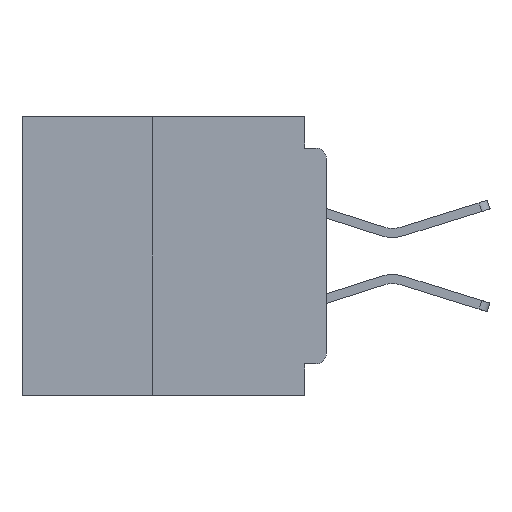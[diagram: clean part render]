
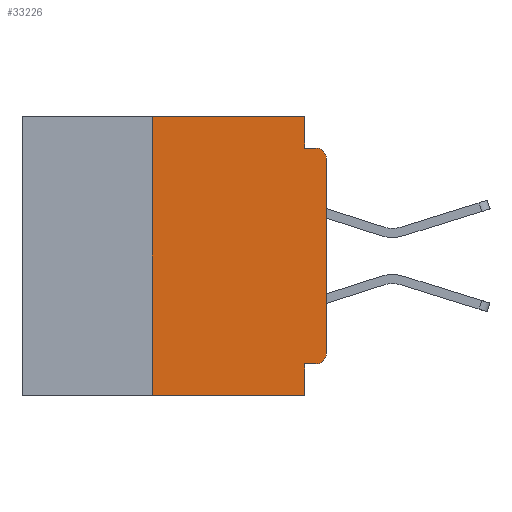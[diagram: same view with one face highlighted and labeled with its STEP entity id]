
A CAD part, left-side view. The second image highlights one B-rep face of the part: STEP entity #33226.
In plain terms, the highlighted planar face has unit normal (-1, 0, 0).
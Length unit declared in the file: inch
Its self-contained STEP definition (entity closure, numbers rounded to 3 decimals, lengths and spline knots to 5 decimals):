
#401 = DIRECTION ( 'NONE',  ( 0., -1., 0. ) ) ;
#425 = CARTESIAN_POINT ( 'NONE',  ( 0., 0., -0.06 ) ) ;
#578 = ORIENTED_EDGE ( 'NONE', *, *, #38165, .F. ) ;
#789 = VECTOR ( 'NONE', #48759, 39.37008 ) ;
#852 = VECTOR ( 'NONE', #14999, 39.37008 ) ;
#1643 = CARTESIAN_POINT ( 'NONE',  ( 0., 0.437, 0. ) ) ;
#2049 = CARTESIAN_POINT ( 'NONE',  ( 0., 0.031, -0.4 ) ) ;
#2297 = VECTOR ( 'NONE', #5242, 39.37008 ) ;
#2617 = CIRCLE ( 'NONE', #19181, 0.015 ) ;
#2740 = ORIENTED_EDGE ( 'NONE', *, *, #18805, .F. ) ;
#3304 = VECTOR ( 'NONE', #26643, 39.37008 ) ;
#3781 = LINE ( 'NONE', #22472, #22875 ) ;
#4065 = EDGE_CURVE ( 'NONE', #16272, #38870, #24792, .T. ) ;
#5242 = DIRECTION ( 'NONE',  ( 0., 0., 1. ) ) ;
#5841 = ORIENTED_EDGE ( 'NONE', *, *, #9505, .T. ) ;
#8282 = EDGE_CURVE ( 'NONE', #13142, #38329, #22589, .T. ) ;
#8519 = VERTEX_POINT ( 'NONE', #48036 ) ;
#9505 = EDGE_CURVE ( 'NONE', #8519, #13142, #39668, .T. ) ;
#10257 = VERTEX_POINT ( 'NONE', #2049 ) ;
#11177 = VECTOR ( 'NONE', #35939, 39.37008 ) ;
#11187 = ORIENTED_EDGE ( 'NONE', *, *, #14609, .T. ) ;
#11631 = VERTEX_POINT ( 'NONE', #39704 ) ;
#12135 = VERTEX_POINT ( 'NONE', #31903 ) ;
#12309 = VERTEX_POINT ( 'NONE', #13692 ) ;
#13142 = VERTEX_POINT ( 'NONE', #18499 ) ;
#13692 = CARTESIAN_POINT ( 'NONE',  ( 0., 0.25, -0.4 ) ) ;
#13794 = CARTESIAN_POINT ( 'NONE',  ( 0., 0.015, -0.06 ) ) ;
#14436 = ORIENTED_EDGE ( 'NONE', *, *, #41662, .F. ) ;
#14609 = EDGE_CURVE ( 'NONE', #38329, #15548, #2617, .T. ) ;
#14853 = CARTESIAN_POINT ( 'NONE',  ( 0., 0.031, -0.045 ) ) ;
#14999 = DIRECTION ( 'NONE',  ( 0., 1., 0. ) ) ;
#15255 = ORIENTED_EDGE ( 'NONE', *, *, #32517, .F. ) ;
#15407 = CARTESIAN_POINT ( 'NONE',  ( 0., 0.015, -0.045 ) ) ;
#15548 = VERTEX_POINT ( 'NONE', #15407 ) ;
#15717 = CARTESIAN_POINT ( 'NONE',  ( 0., 0., -0.045 ) ) ;
#16272 = VERTEX_POINT ( 'NONE', #19513 ) ;
#17672 = DIRECTION ( 'NONE',  ( 0., 0., -1. ) ) ;
#18499 = CARTESIAN_POINT ( 'NONE',  ( 0., 0., -0.34 ) ) ;
#18805 = EDGE_CURVE ( 'NONE', #38870, #15548, #45059, .T. ) ;
#19181 = AXIS2_PLACEMENT_3D ( 'NONE', #13794, #40403, #17672 ) ;
#19513 = CARTESIAN_POINT ( 'NONE',  ( 0., 0.031, 0. ) ) ;
#19875 = LINE ( 'NONE', #44783, #789 ) ;
#20286 = DIRECTION ( 'NONE',  ( -1., 0., 0. ) ) ;
#20935 = EDGE_LOOP ( 'NONE', ( #47976, #11187, #2740, #35956, #14436, #578, #30535, #21364, #15255, #5841 ) ) ;
#21364 = ORIENTED_EDGE ( 'NONE', *, *, #33105, .F. ) ;
#21373 = LINE ( 'NONE', #1643, #11177 ) ;
#22472 = CARTESIAN_POINT ( 'NONE',  ( 0., 0.031, -0.4 ) ) ;
#22529 = CARTESIAN_POINT ( 'NONE',  ( 0., 0., -0.355 ) ) ;
#22589 = LINE ( 'NONE', #35703, #2297 ) ;
#22875 = VECTOR ( 'NONE', #41374, 39.37008 ) ;
#23727 = CARTESIAN_POINT ( 'NONE',  ( 0., 0.437, -0.4 ) ) ;
#24792 = LINE ( 'NONE', #26522, #3304 ) ;
#26522 = CARTESIAN_POINT ( 'NONE',  ( 0., 0.031, 0. ) ) ;
#26643 = DIRECTION ( 'NONE',  ( 0., 0., -1. ) ) ;
#27132 = CARTESIAN_POINT ( 'NONE',  ( 0., 0.437, 0. ) ) ;
#27684 = AXIS2_PLACEMENT_3D ( 'NONE', #43004, #20286, #46784 ) ;
#30535 = ORIENTED_EDGE ( 'NONE', *, *, #35635, .T. ) ;
#30951 = PLANE ( 'NONE',  #46803 ) ;
#31903 = CARTESIAN_POINT ( 'NONE',  ( 0., 0.031, -0.355 ) ) ;
#32517 = EDGE_CURVE ( 'NONE', #8519, #12135, #41318, .T. ) ;
#33105 = EDGE_CURVE ( 'NONE', #12135, #10257, #3781, .T. ) ;
#33226 = ADVANCED_FACE ( 'NONE', ( #45950 ), #30951, .F. ) ;
#34751 = DIRECTION ( 'NONE',  ( 0., 0., -1. ) ) ;
#35635 = EDGE_CURVE ( 'NONE', #12309, #10257, #39822, .T. ) ;
#35703 = CARTESIAN_POINT ( 'NONE',  ( 0., 0., 0. ) ) ;
#35939 = DIRECTION ( 'NONE',  ( 0., -1., 0. ) ) ;
#35956 = ORIENTED_EDGE ( 'NONE', *, *, #4065, .F. ) ;
#38165 = EDGE_CURVE ( 'NONE', #12309, #11631, #19875, .T. ) ;
#38329 = VERTEX_POINT ( 'NONE', #425 ) ;
#38870 = VERTEX_POINT ( 'NONE', #14853 ) ;
#39668 = CIRCLE ( 'NONE', #27684, 0.015 ) ;
#39704 = CARTESIAN_POINT ( 'NONE',  ( 0., 0.25, 0. ) ) ;
#39822 = LINE ( 'NONE', #23727, #42182 ) ;
#40403 = DIRECTION ( 'NONE',  ( -1., 0., 0. ) ) ;
#41318 = LINE ( 'NONE', #22529, #852 ) ;
#41374 = DIRECTION ( 'NONE',  ( 0., 0., -1. ) ) ;
#41662 = EDGE_CURVE ( 'NONE', #11631, #16272, #21373, .T. ) ;
#42182 = VECTOR ( 'NONE', #46385, 39.37008 ) ;
#43004 = CARTESIAN_POINT ( 'NONE',  ( 0., 0.015, -0.34 ) ) ;
#44783 = CARTESIAN_POINT ( 'NONE',  ( 0., 0.25, -0.4 ) ) ;
#45059 = LINE ( 'NONE', #15717, #47444 ) ;
#45950 = FACE_OUTER_BOUND ( 'NONE', #20935, .T. ) ;
#45965 = DIRECTION ( 'NONE',  ( 1., 0., 0. ) ) ;
#46385 = DIRECTION ( 'NONE',  ( 0., -1., 0. ) ) ;
#46784 = DIRECTION ( 'NONE',  ( 0., 0., -1. ) ) ;
#46803 = AXIS2_PLACEMENT_3D ( 'NONE', #27132, #45965, #34751 ) ;
#47444 = VECTOR ( 'NONE', #401, 39.37008 ) ;
#47976 = ORIENTED_EDGE ( 'NONE', *, *, #8282, .T. ) ;
#48036 = CARTESIAN_POINT ( 'NONE',  ( 0., 0.015, -0.355 ) ) ;
#48759 = DIRECTION ( 'NONE',  ( 0., 0., 1. ) ) ;
